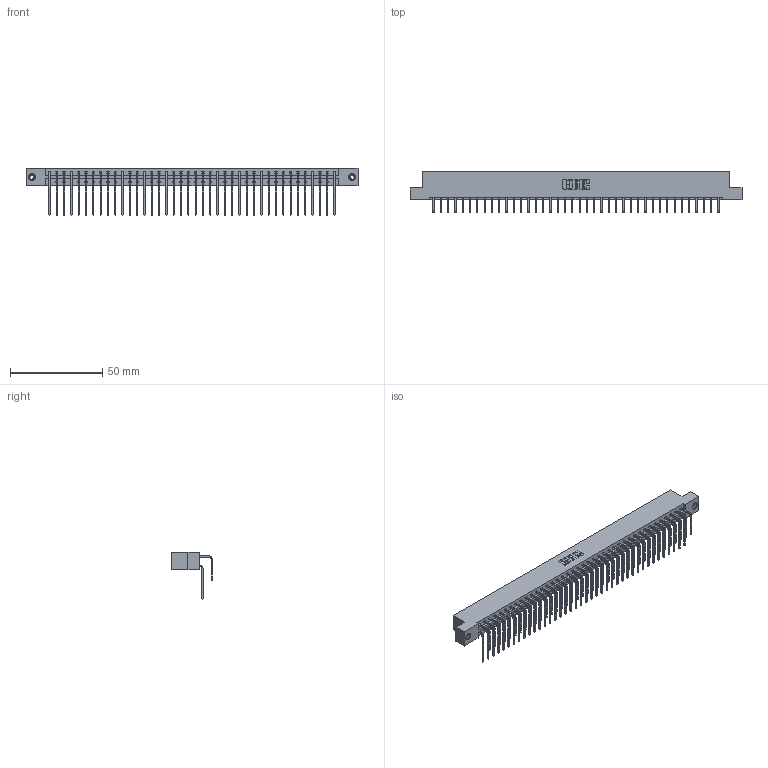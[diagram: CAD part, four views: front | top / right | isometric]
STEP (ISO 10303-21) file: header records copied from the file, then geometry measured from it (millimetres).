
FILE_DESCRIPTION (( 'STEP AP203' ), '1' );
FILE_NAME ('333-080-558-208.STEP', '2018-08-05T02:10:31', ( '' ), ( '' ), 'SwSTEP 2.0', 'SolidWorks 2016', '' );
FILE_SCHEMA (( 'CONFIG_CONTROL_DESIGN' ));
Length unit declared in the file: inch
Products named in the file (5): 333 Part_Flush - .156 Dia - TI; 345-292-001_558 559 Tail - 1; 345-292-001_558 Tail - 2; 345-250-001_345-250-003-102; 333-080-558-208
Assembly tree (83 placements, depth 2):
  333-080-558-208
    333 Part_Flush - .156 Dia - TI
    345-292-001_558 559 Tail - 1  x40
    345-292-001_558 Tail - 2  x40
    345-250-001_345-250-003-102  x2
Bounding box: 180.04 x 22.17 x 25.53 mm (x, y, z)
Volume: 18816.8 mm3; surface area: 24545.2 mm2
Topology: 83 solids, 83 shells, 4494 faces, 13327 edges, 8770 vertices
Faces by surface type: plane 3142, cylinder 1336, cone 12, torus 4
Entity records: 28962 total; most frequent: CARTESIAN_POINT 4836, ORIENTED_EDGE 4714, DIRECTION 4147, EDGE_CURVE 2357, LINE 2169, VECTOR 2169, VERTEX_POINT 1564, AXIS2_PLACEMENT_3D 989
